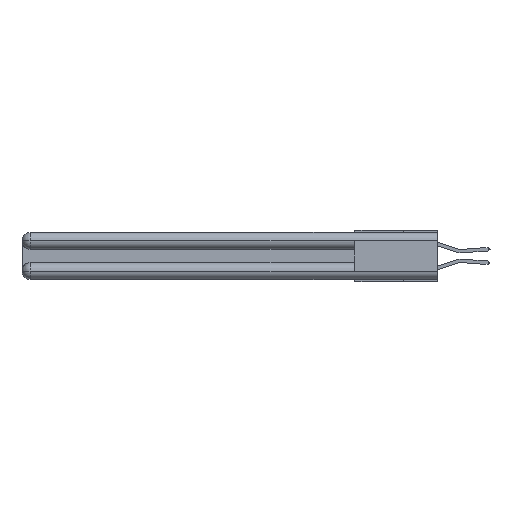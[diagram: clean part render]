
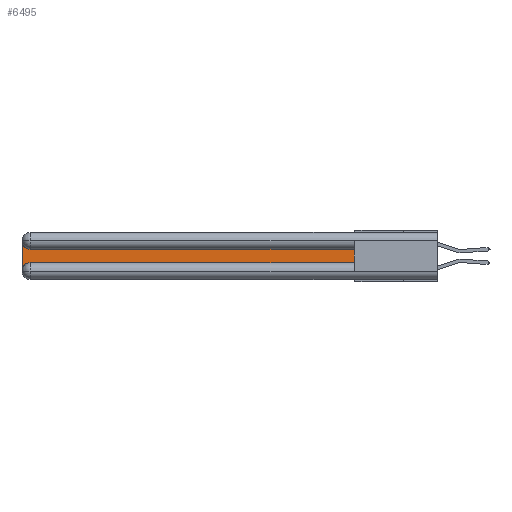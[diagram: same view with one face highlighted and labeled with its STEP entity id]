
A CAD part, left-side view. The second image highlights one B-rep face of the part: STEP entity #6495.
In plain terms, the highlighted planar face has unit normal (-1, 0, 0).
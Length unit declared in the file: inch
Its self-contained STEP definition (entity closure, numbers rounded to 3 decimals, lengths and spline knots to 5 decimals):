
#510 = VERTEX_POINT ( 'NONE', #16601 ) ;
#895 = VERTEX_POINT ( 'NONE', #4075 ) ;
#1532 = PLANE ( 'NONE',  #18595 ) ;
#2166 = ORIENTED_EDGE ( 'NONE', *, *, #28433, .T. ) ;
#2567 = LINE ( 'NONE', #9517, #28956 ) ;
#2845 = CARTESIAN_POINT ( 'NONE',  ( 0.075, 2.94, -0.0625 ) ) ;
#3142 = CIRCLE ( 'NONE', #18285, 0.06 ) ;
#3295 = DIRECTION ( 'NONE',  ( 0., 0., -1. ) ) ;
#3927 = CARTESIAN_POINT ( 'NONE',  ( 0.075, 3., -0.1225 ) ) ;
#4037 = DIRECTION ( 'NONE',  ( 1., 0., 0. ) ) ;
#4075 = CARTESIAN_POINT ( 'NONE',  ( 0.075, 2.94, -0.2175 ) ) ;
#5439 = ORIENTED_EDGE ( 'NONE', *, *, #25660, .T. ) ;
#6159 = CARTESIAN_POINT ( 'NONE',  ( 0.075, 3., -0.0625 ) ) ;
#6240 = CARTESIAN_POINT ( 'NONE',  ( 0.075, 0.6, -0.2175 ) ) ;
#6495 = ADVANCED_FACE ( 'NONE', ( #7356 ), #1532, .F. ) ;
#6745 = LINE ( 'NONE', #30791, #7507 ) ;
#7356 = FACE_OUTER_BOUND ( 'NONE', #24114, .T. ) ;
#7507 = VECTOR ( 'NONE', #30363, 39.37008 ) ;
#7780 = DIRECTION ( 'NONE',  ( 1., 0., 0. ) ) ;
#8179 = CARTESIAN_POINT ( 'NONE',  ( 0.075, 3., -0.2175 ) ) ;
#8524 = EDGE_CURVE ( 'NONE', #19113, #510, #22392, .T. ) ;
#8933 = EDGE_CURVE ( 'NONE', #31944, #22819, #2567, .T. ) ;
#9209 = VERTEX_POINT ( 'NONE', #9279 ) ;
#9279 = CARTESIAN_POINT ( 'NONE',  ( 0.075, 2.94, -0.1225 ) ) ;
#9344 = CIRCLE ( 'NONE', #12848, 0.06 ) ;
#9517 = CARTESIAN_POINT ( 'NONE',  ( 0.075, 0.6, -0.2175 ) ) ;
#10096 = LINE ( 'NONE', #16881, #22953 ) ;
#10612 = DIRECTION ( 'NONE',  ( 1., 0., 0. ) ) ;
#12073 = ORIENTED_EDGE ( 'NONE', *, *, #17491, .T. ) ;
#12848 = AXIS2_PLACEMENT_3D ( 'NONE', #22712, #10612, #3295 ) ;
#16019 = DIRECTION ( 'NONE',  ( 0., 0., -1. ) ) ;
#16601 = CARTESIAN_POINT ( 'NONE',  ( 0.075, 3., -0.2775 ) ) ;
#16694 = EDGE_CURVE ( 'NONE', #510, #895, #9344, .T. ) ;
#16881 = CARTESIAN_POINT ( 'NONE',  ( 0.075, 0.6, -0.1225 ) ) ;
#17491 = EDGE_CURVE ( 'NONE', #22819, #9209, #10096, .T. ) ;
#18141 = ORIENTED_EDGE ( 'NONE', *, *, #16694, .T. ) ;
#18285 = AXIS2_PLACEMENT_3D ( 'NONE', #2845, #7780, #29607 ) ;
#18595 = AXIS2_PLACEMENT_3D ( 'NONE', #3927, #4037, #18998 ) ;
#18998 = DIRECTION ( 'NONE',  ( 0., 0., -1. ) ) ;
#19113 = VERTEX_POINT ( 'NONE', #6159 ) ;
#22349 = DIRECTION ( 'NONE',  ( 0., 0., 1. ) ) ;
#22392 = LINE ( 'NONE', #8179, #28203 ) ;
#22712 = CARTESIAN_POINT ( 'NONE',  ( 0.075, 2.94, -0.2775 ) ) ;
#22819 = VERTEX_POINT ( 'NONE', #26012 ) ;
#22953 = VECTOR ( 'NONE', #27162, 39.37008 ) ;
#23136 = ORIENTED_EDGE ( 'NONE', *, *, #8933, .T. ) ;
#24114 = EDGE_LOOP ( 'NONE', ( #12073, #2166, #30427, #18141, #5439, #23136 ) ) ;
#25660 = EDGE_CURVE ( 'NONE', #895, #31944, #6745, .T. ) ;
#26012 = CARTESIAN_POINT ( 'NONE',  ( 0.075, 0.6, -0.1225 ) ) ;
#27162 = DIRECTION ( 'NONE',  ( 0., 1., 0. ) ) ;
#28203 = VECTOR ( 'NONE', #16019, 39.37008 ) ;
#28433 = EDGE_CURVE ( 'NONE', #9209, #19113, #3142, .T. ) ;
#28956 = VECTOR ( 'NONE', #22349, 39.37008 ) ;
#29607 = DIRECTION ( 'NONE',  ( 0., 0., -1. ) ) ;
#30363 = DIRECTION ( 'NONE',  ( 0., -1., 0. ) ) ;
#30427 = ORIENTED_EDGE ( 'NONE', *, *, #8524, .T. ) ;
#30791 = CARTESIAN_POINT ( 'NONE',  ( 0.075, 0.6, -0.2175 ) ) ;
#31944 = VERTEX_POINT ( 'NONE', #6240 ) ;
